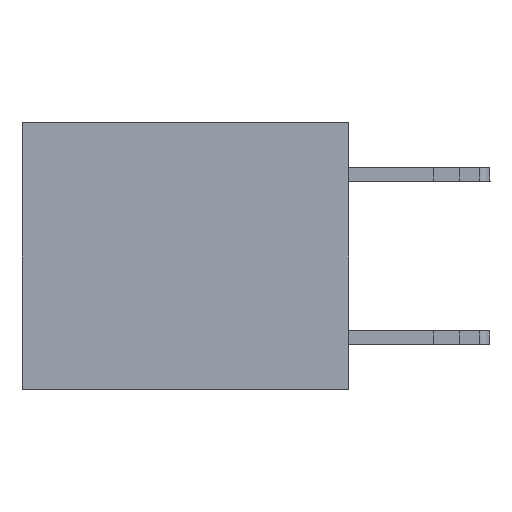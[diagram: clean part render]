
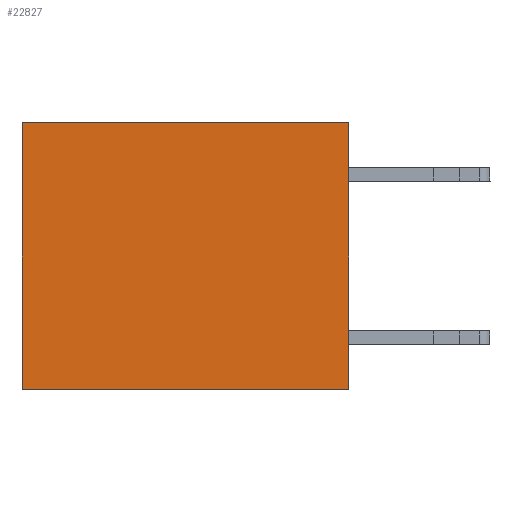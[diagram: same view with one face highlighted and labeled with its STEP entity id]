
A CAD part, left-side view. The second image highlights one B-rep face of the part: STEP entity #22827.
In plain terms, the highlighted planar face has unit normal (-1, 0, 0).
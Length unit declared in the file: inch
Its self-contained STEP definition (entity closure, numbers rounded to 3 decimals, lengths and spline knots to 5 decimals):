
#132 = VECTOR ( 'NONE', #10992, 39.37008 ) ;
#299 = FACE_OUTER_BOUND ( 'NONE', #21454, .T. ) ;
#403 = LINE ( 'NONE', #7064, #132 ) ;
#1339 = VECTOR ( 'NONE', #8572, 39.37008 ) ;
#2945 = DIRECTION ( 'NONE',  ( 0., 1., 0. ) ) ;
#4093 = DIRECTION ( 'NONE',  ( 1., 0., 0. ) ) ;
#4255 = ORIENTED_EDGE ( 'NONE', *, *, #17098, .F. ) ;
#4485 = ORIENTED_EDGE ( 'NONE', *, *, #23395, .T. ) ;
#5686 = EDGE_CURVE ( 'NONE', #17687, #6175, #13597, .T. ) ;
#5763 = PLANE ( 'NONE',  #18979 ) ;
#5898 = CARTESIAN_POINT ( 'NONE',  ( 0.3165, 0.6, 0. ) ) ;
#6175 = VERTEX_POINT ( 'NONE', #5898 ) ;
#7064 = CARTESIAN_POINT ( 'NONE',  ( 0.3165, 0., -0.49 ) ) ;
#7702 = CARTESIAN_POINT ( 'NONE',  ( 0.3165, 0., -0.49 ) ) ;
#7775 = CARTESIAN_POINT ( 'NONE',  ( 0.3165, 0.6, -0.49 ) ) ;
#8572 = DIRECTION ( 'NONE',  ( 0., 1., 0. ) ) ;
#10848 = DIRECTION ( 'NONE',  ( 0., 0., -1. ) ) ;
#10866 = ORIENTED_EDGE ( 'NONE', *, *, #11619, .F. ) ;
#10992 = DIRECTION ( 'NONE',  ( 0., 0., -1. ) ) ;
#11250 = DIRECTION ( 'NONE',  ( 0., 0., -1. ) ) ;
#11448 = VERTEX_POINT ( 'NONE', #7775 ) ;
#11619 = EDGE_CURVE ( 'NONE', #22086, #11448, #20767, .T. ) ;
#12501 = LINE ( 'NONE', #17923, #23349 ) ;
#13597 = LINE ( 'NONE', #23122, #1339 ) ;
#13753 = CARTESIAN_POINT ( 'NONE',  ( 0.3165, 0., 0. ) ) ;
#15459 = CARTESIAN_POINT ( 'NONE',  ( 0.3165, 0., -0.49 ) ) ;
#17098 = EDGE_CURVE ( 'NONE', #17687, #22086, #403, .T. ) ;
#17687 = VERTEX_POINT ( 'NONE', #13753 ) ;
#17923 = CARTESIAN_POINT ( 'NONE',  ( 0.3165, 0.6, -0.49 ) ) ;
#18979 = AXIS2_PLACEMENT_3D ( 'NONE', #7702, #4093, #11250 ) ;
#19543 = ORIENTED_EDGE ( 'NONE', *, *, #5686, .T. ) ;
#20767 = LINE ( 'NONE', #15459, #21899 ) ;
#21454 = EDGE_LOOP ( 'NONE', ( #4485, #10866, #4255, #19543 ) ) ;
#21899 = VECTOR ( 'NONE', #2945, 39.37008 ) ;
#22086 = VERTEX_POINT ( 'NONE', #23399 ) ;
#22827 = ADVANCED_FACE ( 'NONE', ( #299 ), #5763, .F. ) ;
#23122 = CARTESIAN_POINT ( 'NONE',  ( 0.3165, 0., 0. ) ) ;
#23349 = VECTOR ( 'NONE', #10848, 39.37008 ) ;
#23395 = EDGE_CURVE ( 'NONE', #6175, #11448, #12501, .T. ) ;
#23399 = CARTESIAN_POINT ( 'NONE',  ( 0.3165, 0., -0.49 ) ) ;
